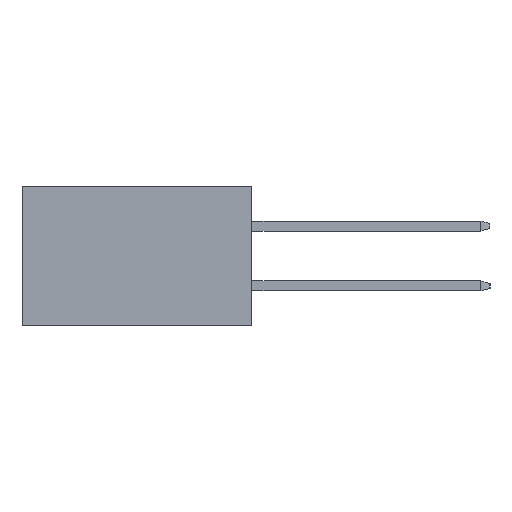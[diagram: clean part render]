
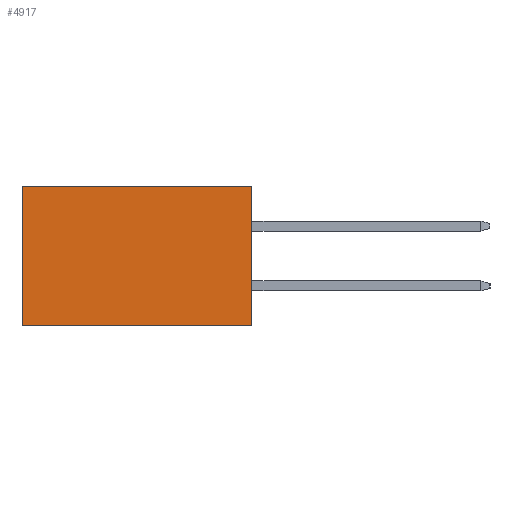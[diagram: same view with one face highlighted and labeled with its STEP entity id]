
A CAD part, left-side view. The second image highlights one B-rep face of the part: STEP entity #4917.
In plain terms, the highlighted planar face has unit normal (-1, 0, 0).
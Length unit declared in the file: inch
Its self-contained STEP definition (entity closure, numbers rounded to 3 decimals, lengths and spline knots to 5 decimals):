
#575 = LINE ( 'NONE', #20578, #21485 ) ;
#1111 = CARTESIAN_POINT ( 'NONE',  ( 0.3205, 0.72, -0.437 ) ) ;
#1145 = VERTEX_POINT ( 'NONE', #18506 ) ;
#2390 = VECTOR ( 'NONE', #12416, 39.37008 ) ;
#2685 = ORIENTED_EDGE ( 'NONE', *, *, #12492, .T. ) ;
#3163 = DIRECTION ( 'NONE',  ( 0., 0., -1. ) ) ;
#3867 = DIRECTION ( 'NONE',  ( 0., 1., 0. ) ) ;
#4063 = VERTEX_POINT ( 'NONE', #12455 ) ;
#4311 = CARTESIAN_POINT ( 'NONE',  ( 0.3205, 0., -0.437 ) ) ;
#4917 = ADVANCED_FACE ( 'NONE', ( #19165 ), #5904, .F. ) ;
#5750 = CARTESIAN_POINT ( 'NONE',  ( 0.3205, 0., 0. ) ) ;
#5904 = PLANE ( 'NONE',  #19221 ) ;
#6367 = CARTESIAN_POINT ( 'NONE',  ( 0.3205, 0.72, -0.437 ) ) ;
#7398 = LINE ( 'NONE', #4311, #13505 ) ;
#7567 = VERTEX_POINT ( 'NONE', #1111 ) ;
#8611 = VECTOR ( 'NONE', #3163, 39.37008 ) ;
#9709 = EDGE_LOOP ( 'NONE', ( #2685, #20015, #18149, #13577 ) ) ;
#10931 = CARTESIAN_POINT ( 'NONE',  ( 0.3205, 0., -0.437 ) ) ;
#12416 = DIRECTION ( 'NONE',  ( 0., 1., 0. ) ) ;
#12455 = CARTESIAN_POINT ( 'NONE',  ( 0.3205, 0.72, 0. ) ) ;
#12492 = EDGE_CURVE ( 'NONE', #4063, #7567, #16568, .T. ) ;
#13505 = VECTOR ( 'NONE', #3867, 39.37008 ) ;
#13577 = ORIENTED_EDGE ( 'NONE', *, *, #20364, .T. ) ;
#14391 = CARTESIAN_POINT ( 'NONE',  ( 0.3205, 0., 0. ) ) ;
#15018 = VERTEX_POINT ( 'NONE', #14391 ) ;
#16568 = LINE ( 'NONE', #6367, #8611 ) ;
#17633 = DIRECTION ( 'NONE',  ( 1., 0., 0. ) ) ;
#18149 = ORIENTED_EDGE ( 'NONE', *, *, #20953, .F. ) ;
#18506 = CARTESIAN_POINT ( 'NONE',  ( 0.3205, 0., -0.437 ) ) ;
#18921 = DIRECTION ( 'NONE',  ( 0., 0., -1. ) ) ;
#19165 = FACE_OUTER_BOUND ( 'NONE', #9709, .T. ) ;
#19221 = AXIS2_PLACEMENT_3D ( 'NONE', #10931, #17633, #20932 ) ;
#19279 = EDGE_CURVE ( 'NONE', #1145, #7567, #7398, .T. ) ;
#20015 = ORIENTED_EDGE ( 'NONE', *, *, #19279, .F. ) ;
#20364 = EDGE_CURVE ( 'NONE', #15018, #4063, #20763, .T. ) ;
#20578 = CARTESIAN_POINT ( 'NONE',  ( 0.3205, 0., -0.437 ) ) ;
#20763 = LINE ( 'NONE', #5750, #2390 ) ;
#20932 = DIRECTION ( 'NONE',  ( 0., 0., -1. ) ) ;
#20953 = EDGE_CURVE ( 'NONE', #15018, #1145, #575, .T. ) ;
#21485 = VECTOR ( 'NONE', #18921, 39.37008 ) ;
